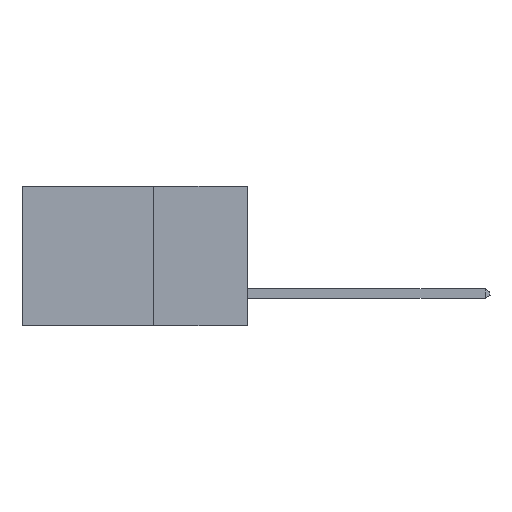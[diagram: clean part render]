
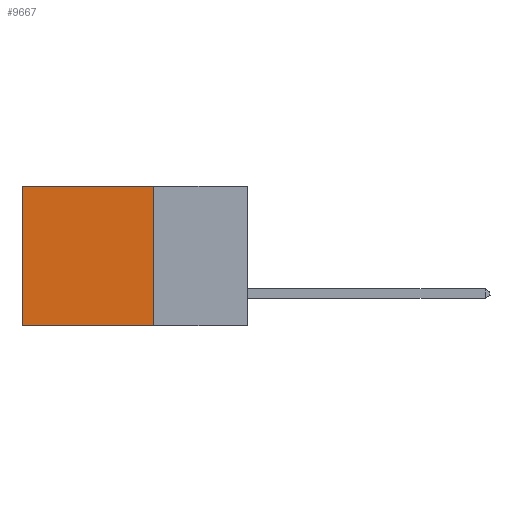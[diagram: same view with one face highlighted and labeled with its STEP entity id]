
A CAD part, left-side view. The second image highlights one B-rep face of the part: STEP entity #9667.
In plain terms, the highlighted planar face has unit normal (-1, 0, 0).
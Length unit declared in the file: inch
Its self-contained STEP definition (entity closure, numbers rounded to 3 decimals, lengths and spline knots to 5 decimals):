
#574 = LINE ( 'NONE', #16124, #1913 ) ;
#709 = EDGE_CURVE ( 'NONE', #12324, #7102, #574, .T. ) ;
#1913 = VECTOR ( 'NONE', #5985, 39.37008 ) ;
#2719 = CARTESIAN_POINT ( 'NONE',  ( 0.298, 0.25, 0. ) ) ;
#2854 = CARTESIAN_POINT ( 'NONE',  ( 0.298, 0.25, -0.37 ) ) ;
#3749 = VECTOR ( 'NONE', #16651, 39.37008 ) ;
#3910 = VECTOR ( 'NONE', #16212, 39.37008 ) ;
#4435 = VERTEX_POINT ( 'NONE', #4666 ) ;
#4666 = CARTESIAN_POINT ( 'NONE',  ( 0.298, 0.25, -0.37 ) ) ;
#5558 = EDGE_LOOP ( 'NONE', ( #20078, #21181, #8213, #9552 ) ) ;
#5985 = DIRECTION ( 'NONE',  ( 0., 0., -1. ) ) ;
#6048 = LINE ( 'NONE', #2719, #3910 ) ;
#7102 = VERTEX_POINT ( 'NONE', #8983 ) ;
#8213 = ORIENTED_EDGE ( 'NONE', *, *, #16562, .F. ) ;
#8370 = PLANE ( 'NONE',  #11159 ) ;
#8545 = LINE ( 'NONE', #9838, #3749 ) ;
#8627 = CARTESIAN_POINT ( 'NONE',  ( 0.298, 0.6, 0. ) ) ;
#8737 = CARTESIAN_POINT ( 'NONE',  ( 0.298, 0.25, 0. ) ) ;
#8983 = CARTESIAN_POINT ( 'NONE',  ( 0.298, 0.6, -0.37 ) ) ;
#9552 = ORIENTED_EDGE ( 'NONE', *, *, #13607, .T. ) ;
#9667 = ADVANCED_FACE ( 'NONE', ( #16471 ), #8370, .F. ) ;
#9838 = CARTESIAN_POINT ( 'NONE',  ( 0.298, 0.25, 0. ) ) ;
#10011 = DIRECTION ( 'NONE',  ( 0., 0., -1. ) ) ;
#11159 = AXIS2_PLACEMENT_3D ( 'NONE', #18393, #13329, #10011 ) ;
#11400 = LINE ( 'NONE', #2854, #16983 ) ;
#11911 = EDGE_CURVE ( 'NONE', #4435, #7102, #11400, .T. ) ;
#12324 = VERTEX_POINT ( 'NONE', #8627 ) ;
#13329 = DIRECTION ( 'NONE',  ( 1., 0., 0. ) ) ;
#13607 = EDGE_CURVE ( 'NONE', #15729, #12324, #6048, .T. ) ;
#15729 = VERTEX_POINT ( 'NONE', #8737 ) ;
#16124 = CARTESIAN_POINT ( 'NONE',  ( 0.298, 0.6, 0. ) ) ;
#16212 = DIRECTION ( 'NONE',  ( 0., 1., 0. ) ) ;
#16471 = FACE_OUTER_BOUND ( 'NONE', #5558, .T. ) ;
#16562 = EDGE_CURVE ( 'NONE', #15729, #4435, #8545, .T. ) ;
#16651 = DIRECTION ( 'NONE',  ( 0., 0., -1. ) ) ;
#16983 = VECTOR ( 'NONE', #17753, 39.37008 ) ;
#17753 = DIRECTION ( 'NONE',  ( 0., 1., 0. ) ) ;
#18393 = CARTESIAN_POINT ( 'NONE',  ( 0.298, 0.25, 0. ) ) ;
#20078 = ORIENTED_EDGE ( 'NONE', *, *, #709, .T. ) ;
#21181 = ORIENTED_EDGE ( 'NONE', *, *, #11911, .F. ) ;
